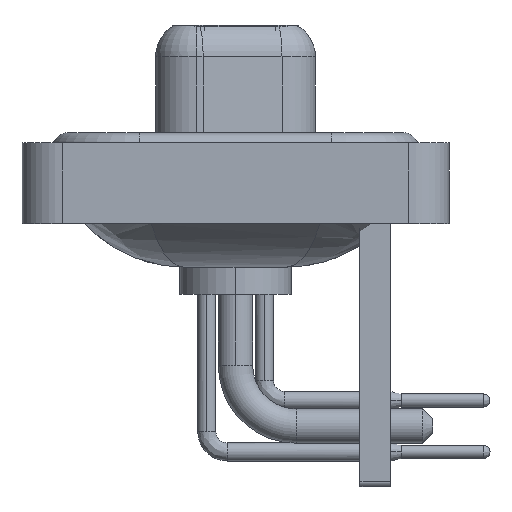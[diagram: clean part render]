
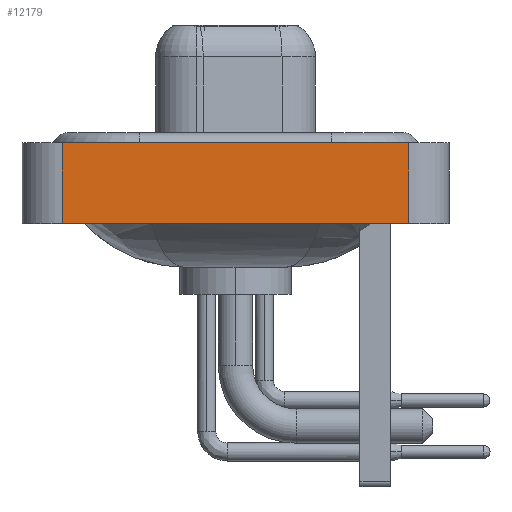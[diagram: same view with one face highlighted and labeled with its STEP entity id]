
A CAD part, left-side view. The second image highlights one B-rep face of the part: STEP entity #12179.
In plain terms, the highlighted planar face has unit normal (-1, 0, 0).
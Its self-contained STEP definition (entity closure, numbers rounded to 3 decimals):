
#863 = DIRECTION ( 'NONE',  ( 0., 0., 1. ) ) ;
#1761 = LINE ( 'NONE', #22063, #10057 ) ;
#1857 = CARTESIAN_POINT ( 'NONE',  ( -7.35, 8.55, -3.6 ) ) ;
#2280 = AXIS2_PLACEMENT_3D ( 'NONE', #12074, #3979, #863 ) ;
#3412 = EDGE_CURVE ( 'NONE', #19199, #9655, #3780, .T. ) ;
#3436 = LINE ( 'NONE', #3774, #19390 ) ;
#3548 = DIRECTION ( 'NONE',  ( 0., -1., 0. ) ) ;
#3771 = DIRECTION ( 'NONE',  ( 0., 0., 1. ) ) ;
#3774 = CARTESIAN_POINT ( 'NONE',  ( -7.35, -8.55, -3.6 ) ) ;
#3780 = LINE ( 'NONE', #12740, #13520 ) ;
#3979 = DIRECTION ( 'NONE',  ( -1., 0., 0. ) ) ;
#4104 = VERTEX_POINT ( 'NONE', #9583 ) ;
#5043 = EDGE_CURVE ( 'NONE', #13434, #19199, #3436, .T. ) ;
#7399 = EDGE_LOOP ( 'NONE', ( #12871, #20294, #23595, #17001 ) ) ;
#7546 = PLANE ( 'NONE',  #2280 ) ;
#7583 = CARTESIAN_POINT ( 'NONE',  ( -7.35, -8.55, 0.4 ) ) ;
#8114 = FACE_OUTER_BOUND ( 'NONE', #7399, .T. ) ;
#8384 = CARTESIAN_POINT ( 'NONE',  ( -7.35, -8.55, 0.4 ) ) ;
#9148 = LINE ( 'NONE', #7583, #13142 ) ;
#9378 = DIRECTION ( 'NONE',  ( 0., 0., 1. ) ) ;
#9448 = EDGE_CURVE ( 'NONE', #13434, #4104, #1761, .T. ) ;
#9583 = CARTESIAN_POINT ( 'NONE',  ( -7.35, 8.55, 0.4 ) ) ;
#9655 = VERTEX_POINT ( 'NONE', #8384 ) ;
#10057 = VECTOR ( 'NONE', #3771, 1000. ) ;
#12074 = CARTESIAN_POINT ( 'NONE',  ( -7.35, -8.55, -3.6 ) ) ;
#12179 = ADVANCED_FACE ( 'NONE', ( #8114 ), #7546, .T. ) ;
#12740 = CARTESIAN_POINT ( 'NONE',  ( -7.35, -8.55, -3.6 ) ) ;
#12871 = ORIENTED_EDGE ( 'NONE', *, *, #3412, .T. ) ;
#13142 = VECTOR ( 'NONE', #16474, 1000. ) ;
#13434 = VERTEX_POINT ( 'NONE', #1857 ) ;
#13520 = VECTOR ( 'NONE', #9378, 1000. ) ;
#14453 = EDGE_CURVE ( 'NONE', #4104, #9655, #9148, .T. ) ;
#16474 = DIRECTION ( 'NONE',  ( 0., -1., 0. ) ) ;
#17001 = ORIENTED_EDGE ( 'NONE', *, *, #5043, .T. ) ;
#19199 = VERTEX_POINT ( 'NONE', #19527 ) ;
#19390 = VECTOR ( 'NONE', #3548, 1000. ) ;
#19527 = CARTESIAN_POINT ( 'NONE',  ( -7.35, -8.55, -3.6 ) ) ;
#20294 = ORIENTED_EDGE ( 'NONE', *, *, #14453, .F. ) ;
#22063 = CARTESIAN_POINT ( 'NONE',  ( -7.35, 8.55, -3.6 ) ) ;
#23595 = ORIENTED_EDGE ( 'NONE', *, *, #9448, .F. ) ;
